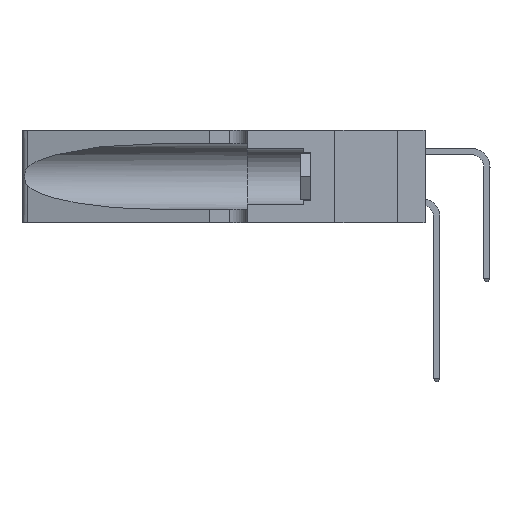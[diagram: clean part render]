
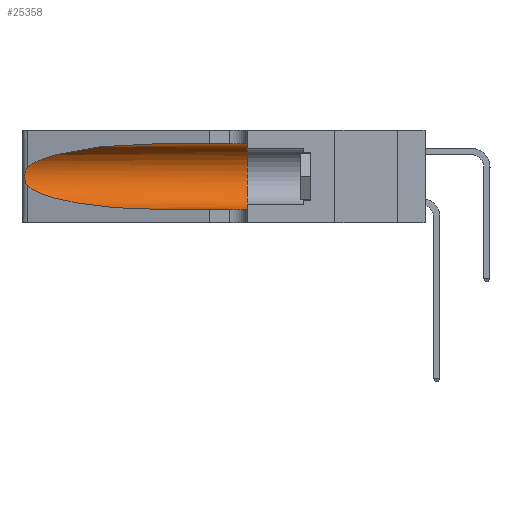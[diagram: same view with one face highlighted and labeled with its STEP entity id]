
A CAD part, left-side view. The second image highlights one B-rep face of the part: STEP entity #25358.
In plain terms, the highlighted cylindrical face has radius 3.308 mm (diameter 6.617 mm), a partial arc.
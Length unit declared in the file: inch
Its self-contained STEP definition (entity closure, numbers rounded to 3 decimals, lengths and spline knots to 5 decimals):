
#682 = B_SPLINE_CURVE_WITH_KNOTS ( 'NONE', 3,
 ( #15361, #26242, #19637, #2145, #17518, #4398, #19727, #6643, #21944, #8861, #24107, #11056, #26337, #13277 ),
 .UNSPECIFIED., .F., .F.,
 ( 4, 2, 2, 2, 2, 2, 4 ),
 ( 0., 0.00027, 0.00053, 0.00107, 0.0016, 0.00187, 0.00214 ),
 .UNSPECIFIED. ) ;
#962 = EDGE_CURVE ( 'NONE', #7966, #5252, #682, .T. ) ;
#1452 = DIRECTION ( 'NONE',  ( 0., -1., 0. ) ) ;
#1609 = CARTESIAN_POINT ( 'NONE',  ( 0.1305, 0.72297, 0.05475 ) ) ;
#1741 = ORIENTED_EDGE ( 'NONE', *, *, #24588, .T. ) ;
#2038 = CARTESIAN_POINT ( 'NONE',  ( 0.1305, 1.61858, 0.05475 ) ) ;
#2145 = CARTESIAN_POINT ( 'NONE',  ( 0.25787, 1.23484, 0.2124 ) ) ;
#2157 = CARTESIAN_POINT ( 'NONE',  ( 0.18966, 0.96281, 0.31525 ) ) ;
#2200 = CARTESIAN_POINT ( 'NONE',  ( 0.1305, 0.35, 0.185 ) ) ;
#2767 = CARTESIAN_POINT ( 'NONE',  ( 0.1305, 0.72297, 0.05475 ) ) ;
#3399 = ORIENTED_EDGE ( 'NONE', *, *, #12491, .F. ) ;
#4027 = CARTESIAN_POINT ( 'NONE',  ( 0.1305, 0.72297, 0.31525 ) ) ;
#4398 = CARTESIAN_POINT ( 'NONE',  ( 0.26018, 1.23835, 0.19895 ) ) ;
#4452 = DIRECTION ( 'NONE',  ( 0., 0., 1. ) ) ;
#4505 = CARTESIAN_POINT ( 'NONE',  ( 0.2373, 1.15595, 0.28018 ) ) ;
#4807 =( BOUNDED_CURVE ( )  B_SPLINE_CURVE ( 3, ( #24609, #26827, #15951, #2767 ),
 .UNSPECIFIED., .F., .T. ) 
 B_SPLINE_CURVE_WITH_KNOTS ( ( 4, 4 ),
 ( 3.44316, 4.71239 ),
 .UNSPECIFIED. ) 
 CURVE ( )  GEOMETRIC_REPRESENTATION_ITEM ( )  RATIONAL_B_SPLINE_CURVE ( ( 1., 0.87, 0.87, 1. ) ) 
 REPRESENTATION_ITEM ( '' )  );
#5239 = VERTEX_POINT ( 'NONE', #1609 ) ;
#5252 = VERTEX_POINT ( 'NONE', #12757 ) ;
#5910 = EDGE_LOOP ( 'NONE', ( #20689, #12905, #1741, #11333, #3399, #13981 ) ) ;
#6633 = EDGE_CURVE ( 'NONE', #5239, #23899, #23278, .T. ) ;
#6643 = CARTESIAN_POINT ( 'NONE',  ( 0.26075, 1.23896, 0.178 ) ) ;
#6648 = CIRCLE ( 'NONE', #27085, 0.13025 ) ;
#6908 = VERTEX_POINT ( 'NONE', #25924 ) ;
#7094 = CARTESIAN_POINT ( 'NONE',  ( 0.1305, 0.35, 0.05475 ) ) ;
#7966 = VERTEX_POINT ( 'NONE', #25000 ) ;
#8247 = EDGE_CURVE ( 'NONE', #10371, #7966, #17104, .T. ) ;
#8861 = CARTESIAN_POINT ( 'NONE',  ( 0.25856, 1.23593, 0.16098 ) ) ;
#10277 = CARTESIAN_POINT ( 'NONE',  ( 0.1305, 0.72297, 0.31525 ) ) ;
#10371 = VERTEX_POINT ( 'NONE', #10277 ) ;
#10958 = DIRECTION ( 'NONE',  ( 0., -1., 0. ) ) ;
#11056 = CARTESIAN_POINT ( 'NONE',  ( 0.25639, 1.23186, 0.15144 ) ) ;
#11333 = ORIENTED_EDGE ( 'NONE', *, *, #6633, .T. ) ;
#11685 = VECTOR ( 'NONE', #10958, 39.37008 ) ;
#12176 = VECTOR ( 'NONE', #1452, 39.37008 ) ;
#12491 = EDGE_CURVE ( 'NONE', #6908, #23899, #6648, .T. ) ;
#12757 = CARTESIAN_POINT ( 'NONE',  ( 0.25487, 1.22718, 0.14631 ) ) ;
#12905 = ORIENTED_EDGE ( 'NONE', *, *, #962, .T. ) ;
#13277 = CARTESIAN_POINT ( 'NONE',  ( 0.25487, 1.22718, 0.14631 ) ) ;
#13981 = ORIENTED_EDGE ( 'NONE', *, *, #22953, .F. ) ;
#15244 = DIRECTION ( 'NONE',  ( 0., 0., -1. ) ) ;
#15361 = CARTESIAN_POINT ( 'NONE',  ( 0.25487, 1.22718, 0.22369 ) ) ;
#15423 = CYLINDRICAL_SURFACE ( 'NONE', #21932, 0.13025 ) ;
#15951 = CARTESIAN_POINT ( 'NONE',  ( 0.18966, 0.96281, 0.05475 ) ) ;
#17104 =( BOUNDED_CURVE ( )  B_SPLINE_CURVE ( 3, ( #4027, #2157, #4505, #19836 ),
 .UNSPECIFIED., .F., .T. ) 
 B_SPLINE_CURVE_WITH_KNOTS ( ( 4, 4 ),
 ( 1.5708, 2.84003 ),
 .UNSPECIFIED. ) 
 CURVE ( )  GEOMETRIC_REPRESENTATION_ITEM ( )  RATIONAL_B_SPLINE_CURVE ( ( 1., 0.87, 0.87, 1. ) ) 
 REPRESENTATION_ITEM ( '' )  );
#17518 = CARTESIAN_POINT ( 'NONE',  ( 0.25854, 1.2359, 0.20912 ) ) ;
#17566 = DIRECTION ( 'NONE',  ( 0., 1., 0. ) ) ;
#19515 = DIRECTION ( 'NONE',  ( 0., -1., 0. ) ) ;
#19637 = CARTESIAN_POINT ( 'NONE',  ( 0.25639, 1.23184, 0.21858 ) ) ;
#19727 = CARTESIAN_POINT ( 'NONE',  ( 0.26075, 1.23896, 0.19203 ) ) ;
#19836 = CARTESIAN_POINT ( 'NONE',  ( 0.25487, 1.22718, 0.22369 ) ) ;
#20689 = ORIENTED_EDGE ( 'NONE', *, *, #8247, .T. ) ;
#21172 = CARTESIAN_POINT ( 'NONE',  ( 0.1305, 1.61858, 0.31525 ) ) ;
#21932 = AXIS2_PLACEMENT_3D ( 'NONE', #28313, #19515, #15244 ) ;
#21944 = CARTESIAN_POINT ( 'NONE',  ( 0.26017, 1.23833, 0.17102 ) ) ;
#22953 = EDGE_CURVE ( 'NONE', #10371, #6908, #24430, .T. ) ;
#23278 = LINE ( 'NONE', #2038, #11685 ) ;
#23899 = VERTEX_POINT ( 'NONE', #7094 ) ;
#24107 = CARTESIAN_POINT ( 'NONE',  ( 0.25789, 1.23486, 0.15765 ) ) ;
#24430 = LINE ( 'NONE', #21172, #12176 ) ;
#24588 = EDGE_CURVE ( 'NONE', #5252, #5239, #4807, .T. ) ;
#24609 = CARTESIAN_POINT ( 'NONE',  ( 0.25487, 1.22718, 0.14631 ) ) ;
#25000 = CARTESIAN_POINT ( 'NONE',  ( 0.25487, 1.22718, 0.22369 ) ) ;
#25358 = ADVANCED_FACE ( 'NONE', ( #27025 ), #15423, .F. ) ;
#25924 = CARTESIAN_POINT ( 'NONE',  ( 0.1305, 0.35, 0.31525 ) ) ;
#26242 = CARTESIAN_POINT ( 'NONE',  ( 0.25555, 1.22994, 0.2215 ) ) ;
#26337 = CARTESIAN_POINT ( 'NONE',  ( 0.25555, 1.22993, 0.14849 ) ) ;
#26827 = CARTESIAN_POINT ( 'NONE',  ( 0.2373, 1.15595, 0.08982 ) ) ;
#27025 = FACE_OUTER_BOUND ( 'NONE', #5910, .T. ) ;
#27085 = AXIS2_PLACEMENT_3D ( 'NONE', #2200, #17566, #4452 ) ;
#28313 = CARTESIAN_POINT ( 'NONE',  ( 0.1305, 1.61858, 0.185 ) ) ;
